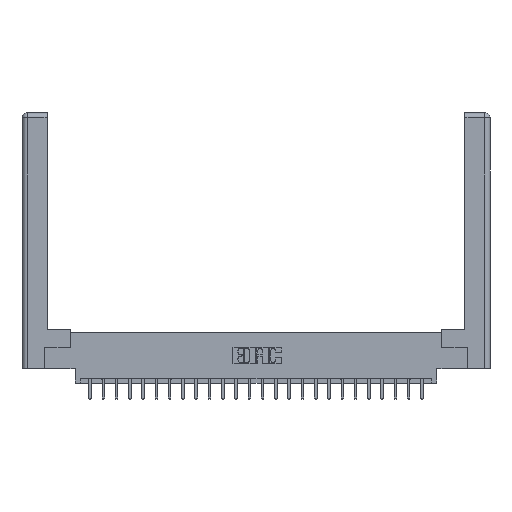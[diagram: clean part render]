
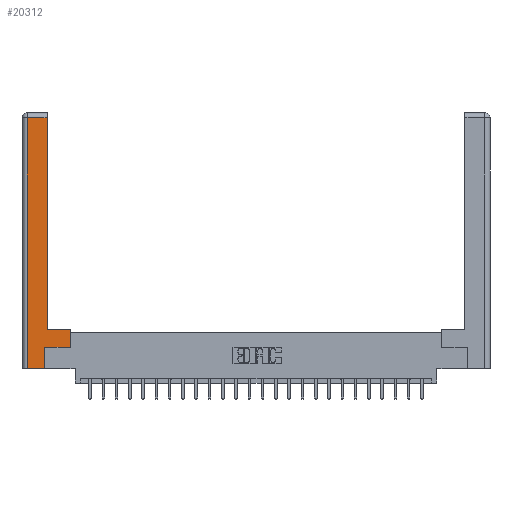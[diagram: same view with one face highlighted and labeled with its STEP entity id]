
A CAD part, top view. The second image highlights one B-rep face of the part: STEP entity #20312.
In plain terms, the highlighted planar face has unit normal (0, 0, 1).
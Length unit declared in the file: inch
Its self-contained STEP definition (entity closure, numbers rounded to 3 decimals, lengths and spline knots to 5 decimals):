
#88 = ORIENTED_EDGE ( 'NONE', *, *, #4900, .T. ) ;
#134 = CARTESIAN_POINT ( 'NONE',  ( 0.565, 0.45, 0. ) ) ;
#520 = PLANE ( 'NONE',  #22007 ) ;
#1943 = LINE ( 'NONE', #17092, #20182 ) ;
#2213 = VECTOR ( 'NONE', #22485, 39.37008 ) ;
#3213 = VECTOR ( 'NONE', #19524, 39.37008 ) ;
#3582 = DIRECTION ( 'NONE',  ( 0., 1., 0. ) ) ;
#3686 = CARTESIAN_POINT ( 'NONE',  ( 0.565, 0.245, 0. ) ) ;
#3885 = ORIENTED_EDGE ( 'NONE', *, *, #21031, .T. ) ;
#4210 = CARTESIAN_POINT ( 'NONE',  ( 0.0615, 0., 0. ) ) ;
#4711 = VERTEX_POINT ( 'NONE', #3686 ) ;
#4900 = EDGE_CURVE ( 'NONE', #11708, #24395, #12491, .T. ) ;
#5468 = CARTESIAN_POINT ( 'NONE',  ( 0.265, 0.245, 0. ) ) ;
#6805 = LINE ( 'NONE', #24921, #16585 ) ;
#7380 = ORIENTED_EDGE ( 'NONE', *, *, #11674, .T. ) ;
#8668 = CARTESIAN_POINT ( 'NONE',  ( 0.0615, 2.94, 0. ) ) ;
#9624 = ORIENTED_EDGE ( 'NONE', *, *, #24522, .T. ) ;
#11095 = EDGE_CURVE ( 'NONE', #15283, #19081, #1943, .T. ) ;
#11674 = EDGE_CURVE ( 'NONE', #24395, #18758, #14034, .T. ) ;
#11708 = VERTEX_POINT ( 'NONE', #20348 ) ;
#11766 = VECTOR ( 'NONE', #20605, 39.37008 ) ;
#12491 = LINE ( 'NONE', #14575, #2213 ) ;
#12617 = LINE ( 'NONE', #13802, #3213 ) ;
#13502 = VERTEX_POINT ( 'NONE', #8668 ) ;
#13708 = CARTESIAN_POINT ( 'NONE',  ( 0.265, 0., 0. ) ) ;
#13720 = EDGE_CURVE ( 'NONE', #4711, #15283, #20937, .T. ) ;
#13802 = CARTESIAN_POINT ( 'NONE',  ( 0.0615, 2.94, 0. ) ) ;
#14034 = LINE ( 'NONE', #22132, #18624 ) ;
#14076 = VERTEX_POINT ( 'NONE', #20151 ) ;
#14575 = CARTESIAN_POINT ( 'NONE',  ( 0.265, 0., 0. ) ) ;
#14932 = ORIENTED_EDGE ( 'NONE', *, *, #19556, .T. ) ;
#15027 = FACE_OUTER_BOUND ( 'NONE', #17162, .T. ) ;
#15283 = VERTEX_POINT ( 'NONE', #134 ) ;
#15569 = LINE ( 'NONE', #15614, #24674 ) ;
#15614 = CARTESIAN_POINT ( 'NONE',  ( 0.565, 0.245, 0. ) ) ;
#15790 = DIRECTION ( 'NONE',  ( 1., 0., 0. ) ) ;
#15797 = ORIENTED_EDGE ( 'NONE', *, *, #11095, .T. ) ;
#16217 = DIRECTION ( 'NONE',  ( 0., 0., -1. ) ) ;
#16282 = ORIENTED_EDGE ( 'NONE', *, *, #18940, .T. ) ;
#16303 = CARTESIAN_POINT ( 'NONE',  ( 0., 0., 0. ) ) ;
#16585 = VECTOR ( 'NONE', #3582, 39.37008 ) ;
#16693 = CARTESIAN_POINT ( 'NONE',  ( 0.565, 0.45, 0. ) ) ;
#17092 = CARTESIAN_POINT ( 'NONE',  ( 0.295, 0.45, 0. ) ) ;
#17162 = EDGE_LOOP ( 'NONE', ( #14932, #16282, #9624, #88, #7380, #3885, #19052, #15797 ) ) ;
#18285 = DIRECTION ( 'NONE',  ( -1., 0., 0. ) ) ;
#18624 = VECTOR ( 'NONE', #24743, 39.37008 ) ;
#18758 = VERTEX_POINT ( 'NONE', #5468 ) ;
#18940 = EDGE_CURVE ( 'NONE', #14076, #13502, #12617, .T. ) ;
#19052 = ORIENTED_EDGE ( 'NONE', *, *, #13720, .T. ) ;
#19081 = VERTEX_POINT ( 'NONE', #19942 ) ;
#19524 = DIRECTION ( 'NONE',  ( -1., 0., 0. ) ) ;
#19556 = EDGE_CURVE ( 'NONE', #19081, #14076, #6805, .T. ) ;
#19942 = CARTESIAN_POINT ( 'NONE',  ( 0.295, 0.45, 0. ) ) ;
#20151 = CARTESIAN_POINT ( 'NONE',  ( 0.295, 2.94, 0. ) ) ;
#20182 = VECTOR ( 'NONE', #22784, 39.37008 ) ;
#20312 = ADVANCED_FACE ( 'NONE', ( #15027 ), #520, .F. ) ;
#20348 = CARTESIAN_POINT ( 'NONE',  ( 0.0615, 0., 0. ) ) ;
#20605 = DIRECTION ( 'NONE',  ( 0., 1., 0. ) ) ;
#20937 = LINE ( 'NONE', #16693, #11766 ) ;
#21031 = EDGE_CURVE ( 'NONE', #18758, #4711, #15569, .T. ) ;
#21897 = DIRECTION ( 'NONE',  ( 0., -1., 0. ) ) ;
#22007 = AXIS2_PLACEMENT_3D ( 'NONE', #16303, #16217, #18285 ) ;
#22132 = CARTESIAN_POINT ( 'NONE',  ( 0.265, 0.245, 0. ) ) ;
#22485 = DIRECTION ( 'NONE',  ( 1., 0., 0. ) ) ;
#22784 = DIRECTION ( 'NONE',  ( -1., 0., 0. ) ) ;
#23925 = LINE ( 'NONE', #4210, #24531 ) ;
#24395 = VERTEX_POINT ( 'NONE', #13708 ) ;
#24522 = EDGE_CURVE ( 'NONE', #13502, #11708, #23925, .T. ) ;
#24531 = VECTOR ( 'NONE', #21897, 39.37008 ) ;
#24674 = VECTOR ( 'NONE', #15790, 39.37008 ) ;
#24743 = DIRECTION ( 'NONE',  ( 0., 1., 0. ) ) ;
#24921 = CARTESIAN_POINT ( 'NONE',  ( 0.295, 3., 0. ) ) ;
